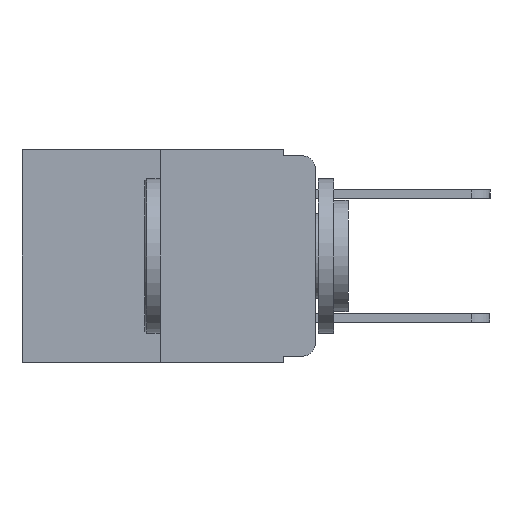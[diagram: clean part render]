
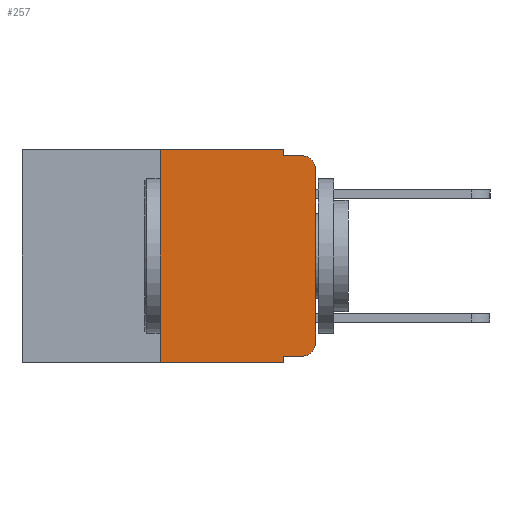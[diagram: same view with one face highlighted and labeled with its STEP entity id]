
A CAD part, left-side view. The second image highlights one B-rep face of the part: STEP entity #257.
In plain terms, the highlighted planar face has unit normal (-1, 0, 0).
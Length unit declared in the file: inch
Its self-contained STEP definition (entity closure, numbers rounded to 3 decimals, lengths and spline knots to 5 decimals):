
#87 = VECTOR ( 'NONE', #6871, 39.37008 ) ;
#257 = ADVANCED_FACE ( 'NONE', ( #3118 ), #3848, .F. ) ;
#288 = EDGE_CURVE ( 'NONE', #3609, #3684, #2815, .T. ) ;
#501 = DIRECTION ( 'NONE',  ( 0., 0., 1. ) ) ;
#520 = CARTESIAN_POINT ( 'NONE',  ( 0., 0.02, -0.01 ) ) ;
#1347 = DIRECTION ( 'NONE',  ( 0., -1., 0. ) ) ;
#1623 = CARTESIAN_POINT ( 'NONE',  ( 0., 0.25, 0. ) ) ;
#1672 = CARTESIAN_POINT ( 'NONE',  ( 0., 0.051, 0. ) ) ;
#1922 = EDGE_CURVE ( 'NONE', #10526, #7870, #4293, .T. ) ;
#1949 = VECTOR ( 'NONE', #10570, 39.37008 ) ;
#1997 = DIRECTION ( 'NONE',  ( 0., -1., 0. ) ) ;
#2085 = LINE ( 'NONE', #3411, #9936 ) ;
#2184 = CARTESIAN_POINT ( 'NONE',  ( 0., 0.051, -0.01 ) ) ;
#2469 = VERTEX_POINT ( 'NONE', #6347 ) ;
#2776 = DIRECTION ( 'NONE',  ( 0., 0., -1. ) ) ;
#2815 = LINE ( 'NONE', #8564, #7692 ) ;
#2847 = LINE ( 'NONE', #6253, #87 ) ;
#3118 = FACE_OUTER_BOUND ( 'NONE', #11215, .T. ) ;
#3319 = CARTESIAN_POINT ( 'NONE',  ( 0., 0.051, -0.333 ) ) ;
#3411 = CARTESIAN_POINT ( 'NONE',  ( 0., 0.473, -0.343 ) ) ;
#3458 = EDGE_CURVE ( 'NONE', #10591, #4791, #9383, .T. ) ;
#3520 = ORIENTED_EDGE ( 'NONE', *, *, #4775, .T. ) ;
#3609 = VERTEX_POINT ( 'NONE', #3319 ) ;
#3684 = VERTEX_POINT ( 'NONE', #6344 ) ;
#3819 = DIRECTION ( 'NONE',  ( 1., 0., 0. ) ) ;
#3848 = PLANE ( 'NONE',  #11504 ) ;
#3870 = DIRECTION ( 'NONE',  ( -1., 0., 0. ) ) ;
#4028 = VERTEX_POINT ( 'NONE', #520 ) ;
#4062 = CARTESIAN_POINT ( 'NONE',  ( 0., 0.473, 0. ) ) ;
#4231 = DIRECTION ( 'NONE',  ( 0., 0., -1. ) ) ;
#4238 = DIRECTION ( 'NONE',  ( -1., 0., 0. ) ) ;
#4260 = CARTESIAN_POINT ( 'NONE',  ( 0., 0.02, -0.313 ) ) ;
#4293 = LINE ( 'NONE', #6180, #1949 ) ;
#4405 = VECTOR ( 'NONE', #12101, 39.37008 ) ;
#4418 = LINE ( 'NONE', #7694, #9390 ) ;
#4775 = EDGE_CURVE ( 'NONE', #3609, #2469, #2847, .T. ) ;
#4791 = VERTEX_POINT ( 'NONE', #10436 ) ;
#4848 = AXIS2_PLACEMENT_3D ( 'NONE', #9509, #3870, #10347 ) ;
#5012 = LINE ( 'NONE', #6532, #9916 ) ;
#5580 = LINE ( 'NONE', #2184, #10397 ) ;
#6063 = EDGE_CURVE ( 'NONE', #4791, #4028, #5580, .T. ) ;
#6180 = CARTESIAN_POINT ( 'NONE',  ( 0., 0., 0. ) ) ;
#6253 = CARTESIAN_POINT ( 'NONE',  ( 0., 0.051, -0.333 ) ) ;
#6344 = CARTESIAN_POINT ( 'NONE',  ( 0., 0.051, -0.343 ) ) ;
#6347 = CARTESIAN_POINT ( 'NONE',  ( 0., 0.02, -0.333 ) ) ;
#6532 = CARTESIAN_POINT ( 'NONE',  ( 0., 0.25, 0. ) ) ;
#6746 = CARTESIAN_POINT ( 'NONE',  ( 0., 0.051, 0. ) ) ;
#6871 = DIRECTION ( 'NONE',  ( 0., -1., 0. ) ) ;
#7306 = VERTEX_POINT ( 'NONE', #7951 ) ;
#7310 = ORIENTED_EDGE ( 'NONE', *, *, #1922, .T. ) ;
#7495 = CIRCLE ( 'NONE', #4848, 0.02 ) ;
#7646 = EDGE_CURVE ( 'NONE', #2469, #10526, #11766, .T. ) ;
#7692 = VECTOR ( 'NONE', #8592, 39.37008 ) ;
#7694 = CARTESIAN_POINT ( 'NONE',  ( 0., 0.473, 0. ) ) ;
#7751 = ORIENTED_EDGE ( 'NONE', *, *, #8999, .T. ) ;
#7870 = VERTEX_POINT ( 'NONE', #8910 ) ;
#7914 = ORIENTED_EDGE ( 'NONE', *, *, #6063, .F. ) ;
#7951 = CARTESIAN_POINT ( 'NONE',  ( 0., 0.25, -0.343 ) ) ;
#8564 = CARTESIAN_POINT ( 'NONE',  ( 0., 0.051, 0. ) ) ;
#8592 = DIRECTION ( 'NONE',  ( 0., 0., -1. ) ) ;
#8727 = ORIENTED_EDGE ( 'NONE', *, *, #3458, .F. ) ;
#8910 = CARTESIAN_POINT ( 'NONE',  ( 0., 0., -0.03 ) ) ;
#8999 = EDGE_CURVE ( 'NONE', #7870, #4028, #7495, .T. ) ;
#9122 = ORIENTED_EDGE ( 'NONE', *, *, #11288, .F. ) ;
#9277 = ORIENTED_EDGE ( 'NONE', *, *, #11613, .F. ) ;
#9383 = LINE ( 'NONE', #6746, #4405 ) ;
#9390 = VECTOR ( 'NONE', #11917, 39.37008 ) ;
#9509 = CARTESIAN_POINT ( 'NONE',  ( 0., 0.02, -0.03 ) ) ;
#9837 = ORIENTED_EDGE ( 'NONE', *, *, #10447, .T. ) ;
#9916 = VECTOR ( 'NONE', #501, 39.37008 ) ;
#9936 = VECTOR ( 'NONE', #1347, 39.37008 ) ;
#9954 = ORIENTED_EDGE ( 'NONE', *, *, #288, .F. ) ;
#10110 = CARTESIAN_POINT ( 'NONE',  ( 0., 0., -0.313 ) ) ;
#10347 = DIRECTION ( 'NONE',  ( 0., 0., -1. ) ) ;
#10397 = VECTOR ( 'NONE', #1997, 39.37008 ) ;
#10436 = CARTESIAN_POINT ( 'NONE',  ( 0., 0.051, -0.01 ) ) ;
#10447 = EDGE_CURVE ( 'NONE', #7306, #3684, #2085, .T. ) ;
#10526 = VERTEX_POINT ( 'NONE', #10110 ) ;
#10548 = ORIENTED_EDGE ( 'NONE', *, *, #7646, .T. ) ;
#10550 = VERTEX_POINT ( 'NONE', #1623 ) ;
#10570 = DIRECTION ( 'NONE',  ( 0., 0., 1. ) ) ;
#10591 = VERTEX_POINT ( 'NONE', #1672 ) ;
#11215 = EDGE_LOOP ( 'NONE', ( #7310, #7751, #7914, #8727, #9122, #9277, #9837, #9954, #3520, #10548 ) ) ;
#11288 = EDGE_CURVE ( 'NONE', #10550, #10591, #4418, .T. ) ;
#11504 = AXIS2_PLACEMENT_3D ( 'NONE', #4062, #3819, #2776 ) ;
#11613 = EDGE_CURVE ( 'NONE', #7306, #10550, #5012, .T. ) ;
#11766 = CIRCLE ( 'NONE', #12089, 0.02 ) ;
#11917 = DIRECTION ( 'NONE',  ( 0., -1., 0. ) ) ;
#12089 = AXIS2_PLACEMENT_3D ( 'NONE', #4260, #4238, #4231 ) ;
#12101 = DIRECTION ( 'NONE',  ( 0., 0., -1. ) ) ;
